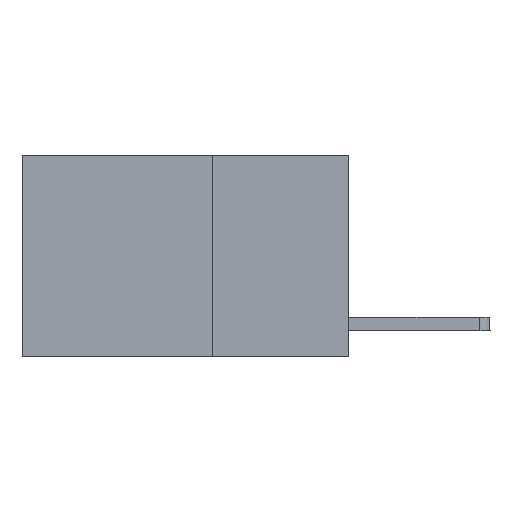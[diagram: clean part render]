
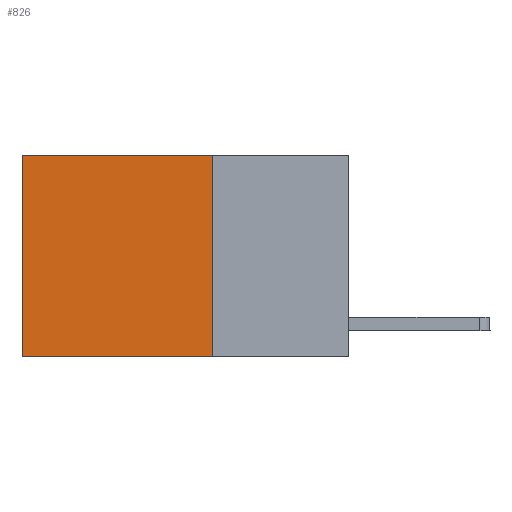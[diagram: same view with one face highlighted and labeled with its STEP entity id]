
A CAD part, left-side view. The second image highlights one B-rep face of the part: STEP entity #826.
In plain terms, the highlighted planar face has unit normal (-1, 0, 0).
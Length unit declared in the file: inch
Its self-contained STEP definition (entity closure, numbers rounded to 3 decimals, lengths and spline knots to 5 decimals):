
#47 = FACE_OUTER_BOUND ( 'NONE', #549, .T. ) ;
#54 = VECTOR ( 'NONE', #9374, 39.37008 ) ;
#173 = CARTESIAN_POINT ( 'NONE',  ( 0.2625, 0.25, -0.37 ) ) ;
#549 = EDGE_LOOP ( 'NONE', ( #2552, #8250, #5312, #4728 ) ) ;
#826 = ADVANCED_FACE ( 'NONE', ( #47 ), #9815, .F. ) ;
#1158 = VERTEX_POINT ( 'NONE', #8279 ) ;
#1847 = CARTESIAN_POINT ( 'NONE',  ( 0.2625, 0.25, 0. ) ) ;
#2552 = ORIENTED_EDGE ( 'NONE', *, *, #3908, .T. ) ;
#2600 = VERTEX_POINT ( 'NONE', #7546 ) ;
#3075 = DIRECTION ( 'NONE',  ( 0., 1., 0. ) ) ;
#3554 = LINE ( 'NONE', #7808, #6582 ) ;
#3669 = EDGE_CURVE ( 'NONE', #2600, #9202, #9593, .T. ) ;
#3841 = AXIS2_PLACEMENT_3D ( 'NONE', #1847, #4146, #5620 ) ;
#3890 = VECTOR ( 'NONE', #3075, 39.37008 ) ;
#3908 = EDGE_CURVE ( 'NONE', #5154, #1158, #3554, .T. ) ;
#4140 = EDGE_CURVE ( 'NONE', #2600, #5154, #4820, .T. ) ;
#4146 = DIRECTION ( 'NONE',  ( 1., 0., 0. ) ) ;
#4728 = ORIENTED_EDGE ( 'NONE', *, *, #4140, .T. ) ;
#4820 = LINE ( 'NONE', #7071, #3890 ) ;
#5154 = VERTEX_POINT ( 'NONE', #5867 ) ;
#5294 = EDGE_CURVE ( 'NONE', #9202, #1158, #5341, .T. ) ;
#5312 = ORIENTED_EDGE ( 'NONE', *, *, #3669, .F. ) ;
#5341 = LINE ( 'NONE', #6284, #54 ) ;
#5620 = DIRECTION ( 'NONE',  ( 0., 0., -1. ) ) ;
#5867 = CARTESIAN_POINT ( 'NONE',  ( 0.2625, 0.6, 0. ) ) ;
#6181 = DIRECTION ( 'NONE',  ( 0., 0., -1. ) ) ;
#6284 = CARTESIAN_POINT ( 'NONE',  ( 0.2625, 0.25, -0.37 ) ) ;
#6582 = VECTOR ( 'NONE', #6181, 39.37008 ) ;
#7071 = CARTESIAN_POINT ( 'NONE',  ( 0.2625, 0.25, 0. ) ) ;
#7373 = VECTOR ( 'NONE', #9699, 39.37008 ) ;
#7546 = CARTESIAN_POINT ( 'NONE',  ( 0.2625, 0.25, 0. ) ) ;
#7808 = CARTESIAN_POINT ( 'NONE',  ( 0.2625, 0.6, 0. ) ) ;
#8250 = ORIENTED_EDGE ( 'NONE', *, *, #5294, .F. ) ;
#8279 = CARTESIAN_POINT ( 'NONE',  ( 0.2625, 0.6, -0.37 ) ) ;
#9202 = VERTEX_POINT ( 'NONE', #173 ) ;
#9374 = DIRECTION ( 'NONE',  ( 0., 1., 0. ) ) ;
#9494 = CARTESIAN_POINT ( 'NONE',  ( 0.2625, 0.25, 0. ) ) ;
#9593 = LINE ( 'NONE', #9494, #7373 ) ;
#9699 = DIRECTION ( 'NONE',  ( 0., 0., -1. ) ) ;
#9815 = PLANE ( 'NONE',  #3841 ) ;
